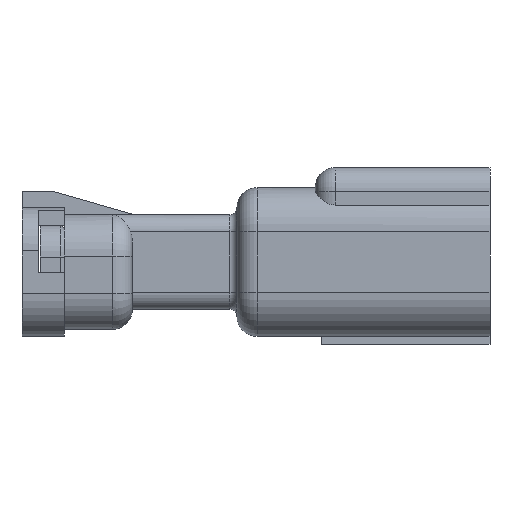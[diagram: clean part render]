
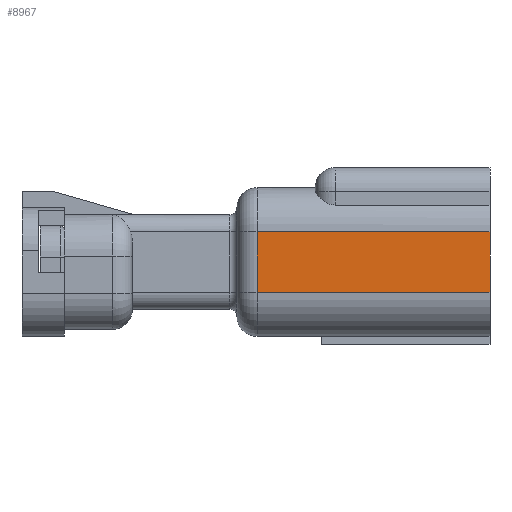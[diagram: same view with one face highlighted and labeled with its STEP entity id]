
A CAD part, left-side view. The second image highlights one B-rep face of the part: STEP entity #8967.
In plain terms, the highlighted planar face has unit normal (-1, 0, 0).
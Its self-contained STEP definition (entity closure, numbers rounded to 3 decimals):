
#290 = DIRECTION ( 'NONE',  ( 0., 1., 0. ) ) ;
#593 = CARTESIAN_POINT ( 'NONE',  ( 3.93, 1.545, 15.944 ) ) ;
#667 = ORIENTED_EDGE ( 'NONE', *, *, #1653, .T. ) ;
#1053 = VECTOR ( 'NONE', #1979, 1000. ) ;
#1059 = VERTEX_POINT ( 'NONE', #12902 ) ;
#1653 = EDGE_CURVE ( 'NONE', #10508, #12440, #17544, .T. ) ;
#1979 = DIRECTION ( 'NONE',  ( 0., -1., 0. ) ) ;
#2514 = ORIENTED_EDGE ( 'NONE', *, *, #8398, .T. ) ;
#2599 = DIRECTION ( 'NONE',  ( 0., 0., 1. ) ) ;
#2659 = CARTESIAN_POINT ( 'NONE',  ( 3.93, 13.145, 15.944 ) ) ;
#3076 = VERTEX_POINT ( 'NONE', #2659 ) ;
#3207 = VECTOR ( 'NONE', #290, 1000. ) ;
#3887 = ORIENTED_EDGE ( 'NONE', *, *, #10906, .T. ) ;
#5505 = CARTESIAN_POINT ( 'NONE',  ( 3.93, 13.145, 15.944 ) ) ;
#5601 = CARTESIAN_POINT ( 'NONE',  ( 3.93, 14.145, 18.944 ) ) ;
#7820 = VECTOR ( 'NONE', #2599, 1000. ) ;
#8181 = LINE ( 'NONE', #5601, #3207 ) ;
#8398 = EDGE_CURVE ( 'NONE', #3076, #10508, #15599, .T. ) ;
#8967 = ADVANCED_FACE ( 'NONE', ( #17257 ), #15662, .F. ) ;
#10508 = VERTEX_POINT ( 'NONE', #593 ) ;
#10521 = CARTESIAN_POINT ( 'NONE',  ( 3.93, 14.145, 13.744 ) ) ;
#10804 = CARTESIAN_POINT ( 'NONE',  ( 3.93, 1.545, 13.744 ) ) ;
#10906 = EDGE_CURVE ( 'NONE', #1059, #3076, #13443, .T. ) ;
#11039 = VECTOR ( 'NONE', #15147, 1000. ) ;
#11089 = CARTESIAN_POINT ( 'NONE',  ( 3.93, 14.145, 15.944 ) ) ;
#11810 = CARTESIAN_POINT ( 'NONE',  ( 3.93, 1.545, 18.944 ) ) ;
#11866 = DIRECTION ( 'NONE',  ( 1., 0., 0. ) ) ;
#12440 = VERTEX_POINT ( 'NONE', #11810 ) ;
#12902 = CARTESIAN_POINT ( 'NONE',  ( 3.93, 13.145, 18.944 ) ) ;
#13443 = LINE ( 'NONE', #5505, #11039 ) ;
#14396 = DIRECTION ( 'NONE',  ( 0., 0., -1. ) ) ;
#15147 = DIRECTION ( 'NONE',  ( 0., 0., -1. ) ) ;
#15281 = EDGE_CURVE ( 'NONE', #12440, #1059, #8181, .T. ) ;
#15599 = LINE ( 'NONE', #11089, #1053 ) ;
#15662 = PLANE ( 'NONE',  #15717 ) ;
#15717 = AXIS2_PLACEMENT_3D ( 'NONE', #10521, #11866, #14396 ) ;
#16678 = EDGE_LOOP ( 'NONE', ( #17483, #3887, #2514, #667 ) ) ;
#17257 = FACE_OUTER_BOUND ( 'NONE', #16678, .T. ) ;
#17483 = ORIENTED_EDGE ( 'NONE', *, *, #15281, .T. ) ;
#17544 = LINE ( 'NONE', #10804, #7820 ) ;
